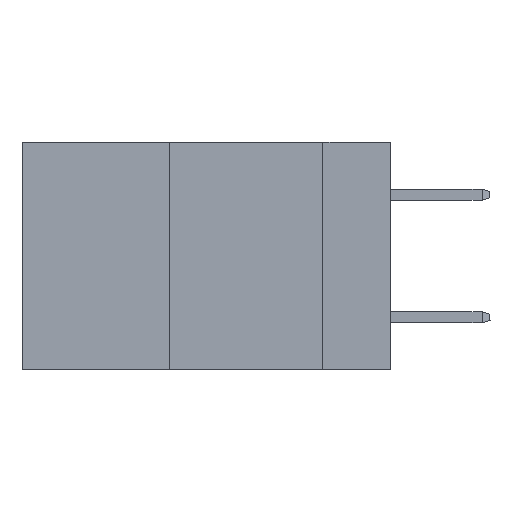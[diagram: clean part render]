
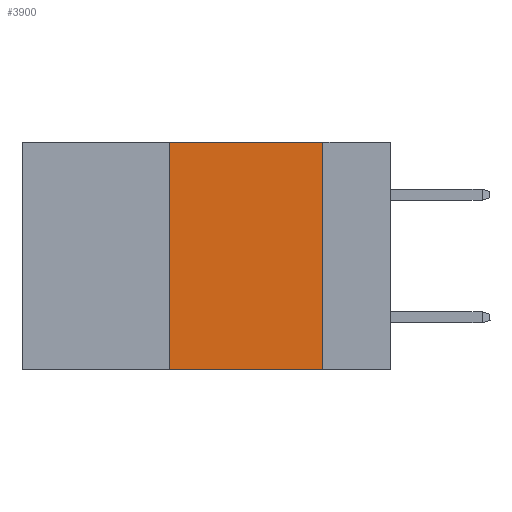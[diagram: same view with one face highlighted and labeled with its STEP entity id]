
A CAD part, left-side view. The second image highlights one B-rep face of the part: STEP entity #3900.
In plain terms, the highlighted planar face has unit normal (-1, 0, 0).
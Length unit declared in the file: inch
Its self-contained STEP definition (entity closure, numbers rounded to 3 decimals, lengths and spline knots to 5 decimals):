
#137 = EDGE_CURVE ( 'NONE', #13584, #751, #14031, .T. ) ;
#751 = VERTEX_POINT ( 'NONE', #7991 ) ;
#1460 = VERTEX_POINT ( 'NONE', #6377 ) ;
#1640 = CARTESIAN_POINT ( 'NONE',  ( 0., 0.6, 0. ) ) ;
#2965 = DIRECTION ( 'NONE',  ( 0., 0., -1. ) ) ;
#3306 = CARTESIAN_POINT ( 'NONE',  ( 0., 0.11, 0. ) ) ;
#3900 = ADVANCED_FACE ( 'NONE', ( #6663 ), #6964, .F. ) ;
#4013 = CARTESIAN_POINT ( 'NONE',  ( 0., 0.36, 0. ) ) ;
#4088 = AXIS2_PLACEMENT_3D ( 'NONE', #1640, #21961, #24280 ) ;
#4877 = ORIENTED_EDGE ( 'NONE', *, *, #22282, .F. ) ;
#5261 = VECTOR ( 'NONE', #2965, 39.37008 ) ;
#6096 = LINE ( 'NONE', #14438, #27611 ) ;
#6377 = CARTESIAN_POINT ( 'NONE',  ( 0., 0.11, 0. ) ) ;
#6663 = FACE_OUTER_BOUND ( 'NONE', #21387, .T. ) ;
#6964 = PLANE ( 'NONE',  #4088 ) ;
#7837 = CARTESIAN_POINT ( 'NONE',  ( 0., 0.6, -0.37 ) ) ;
#7991 = CARTESIAN_POINT ( 'NONE',  ( 0., 0.11, -0.37 ) ) ;
#8057 = VECTOR ( 'NONE', #27103, 39.37008 ) ;
#11437 = ORIENTED_EDGE ( 'NONE', *, *, #26791, .F. ) ;
#12556 = DIRECTION ( 'NONE',  ( 0., -1., 0. ) ) ;
#13584 = VERTEX_POINT ( 'NONE', #22519 ) ;
#14031 = LINE ( 'NONE', #7837, #8057 ) ;
#14438 = CARTESIAN_POINT ( 'NONE',  ( 0., 0.36, 0. ) ) ;
#15341 = ORIENTED_EDGE ( 'NONE', *, *, #21739, .F. ) ;
#15599 = LINE ( 'NONE', #3306, #5261 ) ;
#17448 = CARTESIAN_POINT ( 'NONE',  ( 0., 0.6, 0. ) ) ;
#21387 = EDGE_LOOP ( 'NONE', ( #4877, #11437, #15341, #24182 ) ) ;
#21739 = EDGE_CURVE ( 'NONE', #13584, #32976, #6096, .T. ) ;
#21961 = DIRECTION ( 'NONE',  ( 1., 0., 0. ) ) ;
#22282 = EDGE_CURVE ( 'NONE', #1460, #751, #15599, .T. ) ;
#22519 = CARTESIAN_POINT ( 'NONE',  ( 0., 0.36, -0.37 ) ) ;
#22761 = DIRECTION ( 'NONE',  ( 0., 0., 1. ) ) ;
#23172 = LINE ( 'NONE', #17448, #26335 ) ;
#24182 = ORIENTED_EDGE ( 'NONE', *, *, #137, .T. ) ;
#24280 = DIRECTION ( 'NONE',  ( 0., 0., -1. ) ) ;
#26335 = VECTOR ( 'NONE', #12556, 39.37008 ) ;
#26791 = EDGE_CURVE ( 'NONE', #32976, #1460, #23172, .T. ) ;
#27103 = DIRECTION ( 'NONE',  ( 0., -1., 0. ) ) ;
#27611 = VECTOR ( 'NONE', #22761, 39.37008 ) ;
#32976 = VERTEX_POINT ( 'NONE', #4013 ) ;
